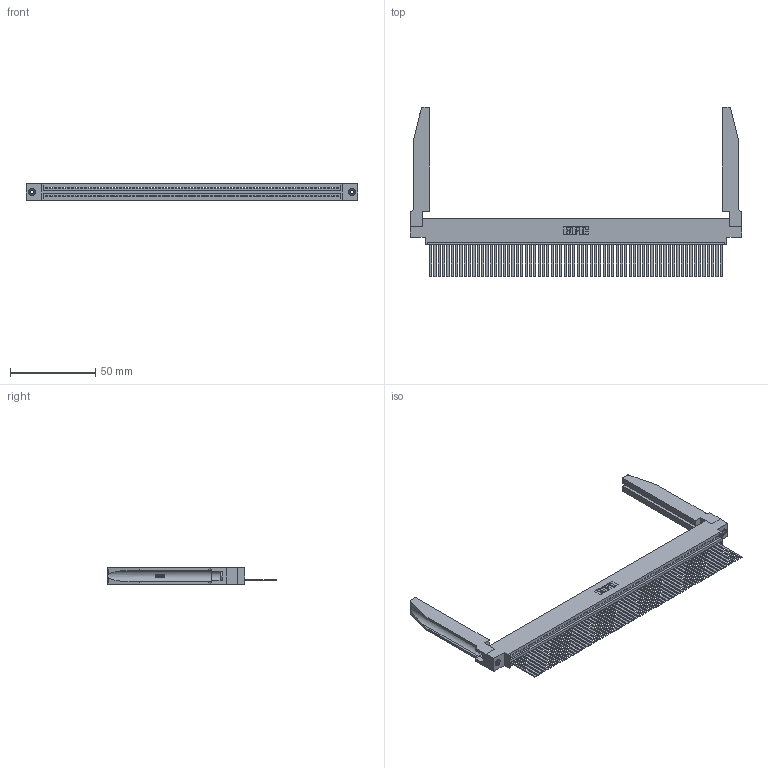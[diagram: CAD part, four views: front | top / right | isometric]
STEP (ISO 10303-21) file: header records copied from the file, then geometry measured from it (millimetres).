
FILE_DESCRIPTION (( 'STEP AP203' ), '1' );
FILE_NAME ('345-068-544-678.STEP', '2019-10-12T08:03:35', ( '' ), ( '' ), 'SwSTEP 2.0', 'SolidWorks 2016', '' );
FILE_SCHEMA (( 'CONFIG_CONTROL_DESIGN' ));
Length unit declared in the file: inch
Products named in the file (5): 345-220-078_345-220-078; 345-068-544-678; 345 Part_0.170 Offset - 0.156 Dia-TH; 345-292-001_345-293-144; 345-250-001_345-250-001-102
Assembly tree (73 placements, depth 2):
  345-068-544-678
    345 Part_0.170 Offset - 0.156 Dia-TH
    345-292-001_345-293-144  x68
    345-250-001_345-250-001-102  x2
    345-220-078_345-220-078  x2
Bounding box: 193.95 x 99.24 x 9.4 mm (x, y, z)
Volume: 27079.6 mm3; surface area: 35349.8 mm2
Topology: 73 solids, 73 shells, 3900 faces, 11705 edges, 7702 vertices
Faces by surface type: plane 2674, cylinder 1174, bspline 36, cone 12, torus 4
Entity records: 52366 total; most frequent: CARTESIAN_POINT 9967, ORIENTED_EDGE 8866, DIRECTION 7671, EDGE_CURVE 4433, VECTOR 3939, LINE 3939, VERTEX_POINT 2948, AXIS2_PLACEMENT_3D 1866
